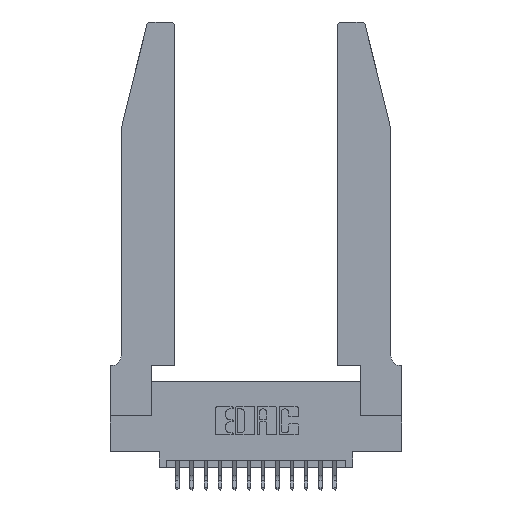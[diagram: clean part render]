
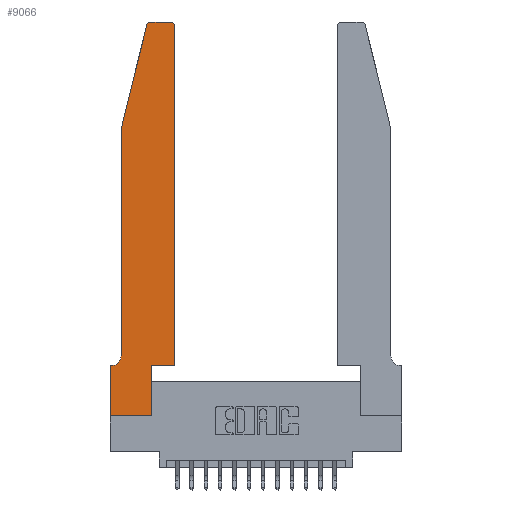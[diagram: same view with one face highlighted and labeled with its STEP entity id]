
A CAD part, top view. The second image highlights one B-rep face of the part: STEP entity #9066.
In plain terms, the highlighted planar face has unit normal (0, 0, 1).
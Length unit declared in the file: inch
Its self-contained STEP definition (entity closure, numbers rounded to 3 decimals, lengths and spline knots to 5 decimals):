
#284 = CARTESIAN_POINT ( 'NONE',  ( 0., 0., 0.37 ) ) ;
#314 = CARTESIAN_POINT ( 'NONE',  ( 0.2605, 2.75, 0.37 ) ) ;
#426 = LINE ( 'NONE', #2673, #9168 ) ;
#571 = CARTESIAN_POINT ( 'NONE',  ( 0.0755, 0.42, 0.37 ) ) ;
#731 = VERTEX_POINT ( 'NONE', #5523 ) ;
#770 = ORIENTED_EDGE ( 'NONE', *, *, #2043, .T. ) ;
#978 = CARTESIAN_POINT ( 'NONE',  ( 0.284, 2.75, 0.37 ) ) ;
#1111 = DIRECTION ( 'NONE',  ( -1., 0., 0. ) ) ;
#1271 = VECTOR ( 'NONE', #16048, 39.37008 ) ;
#1412 = AXIS2_PLACEMENT_3D ( 'NONE', #15365, #3062, #1111 ) ;
#1450 = LINE ( 'NONE', #16270, #8223 ) ;
#1623 = VERTEX_POINT ( 'NONE', #4808 ) ;
#1636 = AXIS2_PLACEMENT_3D ( 'NONE', #11786, #8863, #17562 ) ;
#1742 = CARTESIAN_POINT ( 'NONE',  ( 0.4505, 0.35, 0.37 ) ) ;
#1810 = EDGE_CURVE ( 'NONE', #7831, #12986, #15207, .T. ) ;
#1879 = CARTESIAN_POINT ( 'NONE',  ( 0.4505, 2.72, 0.37 ) ) ;
#1986 = PLANE ( 'NONE',  #18396 ) ;
#2031 = LINE ( 'NONE', #13820, #10811 ) ;
#2043 = EDGE_CURVE ( 'NONE', #731, #7662, #2841, .T. ) ;
#2583 = VECTOR ( 'NONE', #4462, 39.37008 ) ;
#2673 = CARTESIAN_POINT ( 'NONE',  ( 0.0755, 2., 0.37 ) ) ;
#2841 = LINE ( 'NONE', #284, #6459 ) ;
#3037 = EDGE_CURVE ( 'NONE', #5063, #731, #1450, .T. ) ;
#3062 = DIRECTION ( 'NONE',  ( 0., 0., -1. ) ) ;
#3249 = EDGE_CURVE ( 'NONE', #6081, #14637, #12652, .T. ) ;
#3313 = CARTESIAN_POINT ( 'NONE',  ( 0.4205, 2.75, 0.37 ) ) ;
#3356 = ORIENTED_EDGE ( 'NONE', *, *, #4824, .T. ) ;
#3609 = CIRCLE ( 'NONE', #1412, 0.07 ) ;
#3722 = LINE ( 'NONE', #14489, #7534 ) ;
#3979 = VERTEX_POINT ( 'NONE', #8326 ) ;
#4462 = DIRECTION ( 'NONE',  ( 0., -1., 0. ) ) ;
#4566 = EDGE_CURVE ( 'NONE', #1623, #12760, #426, .T. ) ;
#4805 = CARTESIAN_POINT ( 'NONE',  ( 0.2865, 0.35, 0.37 ) ) ;
#4808 = CARTESIAN_POINT ( 'NONE',  ( 0.25487, 2.72718, 0.37 ) ) ;
#4824 = EDGE_CURVE ( 'NONE', #12760, #18535, #6859, .T. ) ;
#5063 = VERTEX_POINT ( 'NONE', #13801 ) ;
#5523 = CARTESIAN_POINT ( 'NONE',  ( 0., 0.35, 0.37 ) ) ;
#5624 = ORIENTED_EDGE ( 'NONE', *, *, #11098, .T. ) ;
#6081 = VERTEX_POINT ( 'NONE', #14956 ) ;
#6341 = CARTESIAN_POINT ( 'NONE',  ( 0.0755, 2., 0.37 ) ) ;
#6427 = AXIS2_PLACEMENT_3D ( 'NONE', #12690, #16822, #9914 ) ;
#6459 = VECTOR ( 'NONE', #14310, 39.37008 ) ;
#6553 = EDGE_CURVE ( 'NONE', #17014, #7831, #15098, .T. ) ;
#6646 = VECTOR ( 'NONE', #9680, 39.37008 ) ;
#6859 = LINE ( 'NONE', #17259, #2583 ) ;
#7095 = CARTESIAN_POINT ( 'NONE',  ( 0., 0., 0.37 ) ) ;
#7534 = VECTOR ( 'NONE', #17197, 39.37008 ) ;
#7544 = DIRECTION ( 'NONE',  ( 0., 1., 0. ) ) ;
#7662 = VERTEX_POINT ( 'NONE', #7095 ) ;
#7831 = VERTEX_POINT ( 'NONE', #3313 ) ;
#8037 = EDGE_CURVE ( 'NONE', #18535, #5063, #3609, .T. ) ;
#8223 = VECTOR ( 'NONE', #17832, 39.37008 ) ;
#8326 = CARTESIAN_POINT ( 'NONE',  ( 0.4505, 0.35, 0.37 ) ) ;
#8438 = DIRECTION ( 'NONE',  ( -0.239, -0.971, 0. ) ) ;
#8648 = ORIENTED_EDGE ( 'NONE', *, *, #16786, .T. ) ;
#8863 = DIRECTION ( 'NONE',  ( 0., 0., 1. ) ) ;
#8953 = DIRECTION ( 'NONE',  ( 1., 0., 0. ) ) ;
#9066 = ADVANCED_FACE ( 'NONE', ( #15665 ), #1986, .T. ) ;
#9168 = VECTOR ( 'NONE', #8438, 39.37008 ) ;
#9641 = DIRECTION ( 'NONE',  ( 1., 0., 0. ) ) ;
#9680 = DIRECTION ( 'NONE',  ( 0., 1., 0. ) ) ;
#9914 = DIRECTION ( 'NONE',  ( 1., 0., 0. ) ) ;
#10380 = ORIENTED_EDGE ( 'NONE', *, *, #1810, .T. ) ;
#10395 = CARTESIAN_POINT ( 'NONE',  ( 0., 0.35, 0.37 ) ) ;
#10396 = ORIENTED_EDGE ( 'NONE', *, *, #8037, .T. ) ;
#10811 = VECTOR ( 'NONE', #9641, 39.37008 ) ;
#11098 = EDGE_CURVE ( 'NONE', #7662, #6081, #3722, .T. ) ;
#11786 = CARTESIAN_POINT ( 'NONE',  ( 0.4205, 2.72, 0.37 ) ) ;
#12135 = CIRCLE ( 'NONE', #6427, 0.03 ) ;
#12412 = EDGE_CURVE ( 'NONE', #12986, #1623, #12135, .T. ) ;
#12652 = LINE ( 'NONE', #15437, #6646 ) ;
#12660 = ORIENTED_EDGE ( 'NONE', *, *, #4566, .T. ) ;
#12690 = CARTESIAN_POINT ( 'NONE',  ( 0.284, 2.72, 0.37 ) ) ;
#12760 = VERTEX_POINT ( 'NONE', #6341 ) ;
#12986 = VERTEX_POINT ( 'NONE', #978 ) ;
#13511 = VECTOR ( 'NONE', #7544, 39.37008 ) ;
#13801 = CARTESIAN_POINT ( 'NONE',  ( 0.0055, 0.35, 0.37 ) ) ;
#13820 = CARTESIAN_POINT ( 'NONE',  ( 0.4505, 0.35, 0.37 ) ) ;
#14310 = DIRECTION ( 'NONE',  ( 0., -1., 0. ) ) ;
#14359 = ORIENTED_EDGE ( 'NONE', *, *, #3037, .T. ) ;
#14489 = CARTESIAN_POINT ( 'NONE',  ( 0., 0., 0.37 ) ) ;
#14635 = ORIENTED_EDGE ( 'NONE', *, *, #3249, .T. ) ;
#14637 = VERTEX_POINT ( 'NONE', #4805 ) ;
#14956 = CARTESIAN_POINT ( 'NONE',  ( 0.2865, 0., 0.37 ) ) ;
#15098 = CIRCLE ( 'NONE', #1636, 0.03 ) ;
#15207 = LINE ( 'NONE', #314, #1271 ) ;
#15365 = CARTESIAN_POINT ( 'NONE',  ( 0.0055, 0.42, 0.37 ) ) ;
#15393 = ORIENTED_EDGE ( 'NONE', *, *, #6553, .T. ) ;
#15437 = CARTESIAN_POINT ( 'NONE',  ( 0.2865, 0.35, 0.37 ) ) ;
#15665 = FACE_OUTER_BOUND ( 'NONE', #18405, .T. ) ;
#16048 = DIRECTION ( 'NONE',  ( -1., 0., 0. ) ) ;
#16228 = DIRECTION ( 'NONE',  ( 0., 0., 1. ) ) ;
#16270 = CARTESIAN_POINT ( 'NONE',  ( 0.0755, 0.35, 0.37 ) ) ;
#16786 = EDGE_CURVE ( 'NONE', #3979, #17014, #17326, .T. ) ;
#16822 = DIRECTION ( 'NONE',  ( 0., 0., 1. ) ) ;
#17014 = VERTEX_POINT ( 'NONE', #1879 ) ;
#17122 = ORIENTED_EDGE ( 'NONE', *, *, #12412, .T. ) ;
#17197 = DIRECTION ( 'NONE',  ( 1., 0., 0. ) ) ;
#17259 = CARTESIAN_POINT ( 'NONE',  ( 0.0755, 2., 0.37 ) ) ;
#17326 = LINE ( 'NONE', #1742, #13511 ) ;
#17562 = DIRECTION ( 'NONE',  ( 1., 0., 0. ) ) ;
#17649 = ORIENTED_EDGE ( 'NONE', *, *, #17694, .T. ) ;
#17694 = EDGE_CURVE ( 'NONE', #14637, #3979, #2031, .T. ) ;
#17832 = DIRECTION ( 'NONE',  ( -1., 0., 0. ) ) ;
#18396 = AXIS2_PLACEMENT_3D ( 'NONE', #10395, #16228, #8953 ) ;
#18405 = EDGE_LOOP ( 'NONE', ( #10380, #17122, #12660, #3356, #10396, #14359, #770, #5624, #14635, #17649, #8648, #15393 ) ) ;
#18535 = VERTEX_POINT ( 'NONE', #571 ) ;
